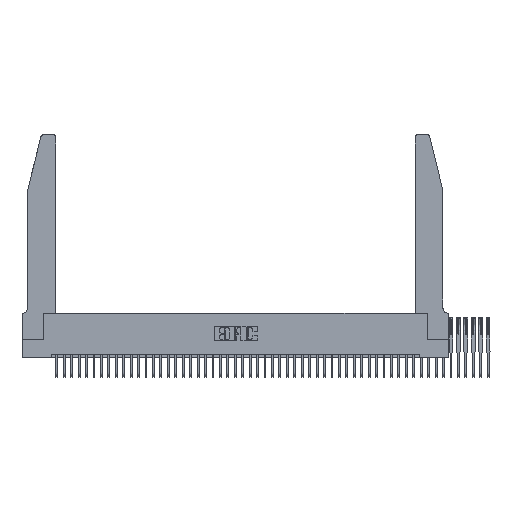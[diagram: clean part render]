
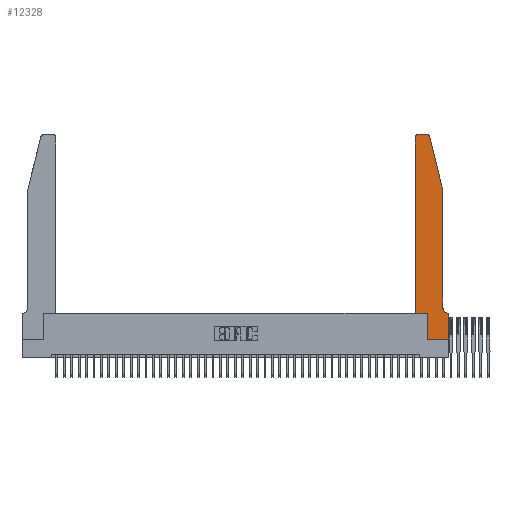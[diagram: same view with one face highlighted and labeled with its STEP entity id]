
A CAD part, top view. The second image highlights one B-rep face of the part: STEP entity #12328.
In plain terms, the highlighted face is planar.
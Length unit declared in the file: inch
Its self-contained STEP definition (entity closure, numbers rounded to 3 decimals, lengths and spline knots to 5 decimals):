
#178 = EDGE_CURVE ( 'NONE', #13072, #494, #8193, .T. ) ;
#361 = CARTESIAN_POINT ( 'NONE',  ( 0.0055, 0.42, 0. ) ) ;
#494 = VERTEX_POINT ( 'NONE', #31878 ) ;
#635 = CARTESIAN_POINT ( 'NONE',  ( 0.25487, 2.72718, 0. ) ) ;
#930 = VECTOR ( 'NONE', #30856, 39.37008 ) ;
#1835 = LINE ( 'NONE', #7803, #26412 ) ;
#2104 = CARTESIAN_POINT ( 'NONE',  ( 0., 0.35, 0. ) ) ;
#2577 = VERTEX_POINT ( 'NONE', #7879 ) ;
#2579 = ORIENTED_EDGE ( 'NONE', *, *, #7124, .F. ) ;
#2732 = CARTESIAN_POINT ( 'NONE',  ( 0.0755, 0.42, 0. ) ) ;
#2834 = EDGE_LOOP ( 'NONE', ( #19985, #33211, #2840, #29865, #11579, #32295, #10594, #4968, #27315, #2579, #9077, #7560 ) ) ;
#2840 = ORIENTED_EDGE ( 'NONE', *, *, #12280, .F. ) ;
#2904 = VERTEX_POINT ( 'NONE', #34921 ) ;
#3621 = DIRECTION ( 'NONE',  ( 0., 0., -1. ) ) ;
#3631 = VECTOR ( 'NONE', #8545, 39.37008 ) ;
#3675 = DIRECTION ( 'NONE',  ( -1., 0., 0. ) ) ;
#4968 = ORIENTED_EDGE ( 'NONE', *, *, #16838, .F. ) ;
#5735 = CARTESIAN_POINT ( 'NONE',  ( 0.2865, 0., 0. ) ) ;
#6922 = VERTEX_POINT ( 'NONE', #35473 ) ;
#7002 = VECTOR ( 'NONE', #38113, 39.37008 ) ;
#7124 = EDGE_CURVE ( 'NONE', #35716, #32932, #27854, .T. ) ;
#7560 = ORIENTED_EDGE ( 'NONE', *, *, #15237, .F. ) ;
#7798 = CIRCLE ( 'NONE', #17933, 0.03 ) ;
#7803 = CARTESIAN_POINT ( 'NONE',  ( 0.2605, 2.75, 0. ) ) ;
#7879 = CARTESIAN_POINT ( 'NONE',  ( 0.4205, 2.75, 0. ) ) ;
#8089 = CARTESIAN_POINT ( 'NONE',  ( 0.0755, 0.35, 0. ) ) ;
#8193 = LINE ( 'NONE', #30409, #32463 ) ;
#8531 = EDGE_CURVE ( 'NONE', #38510, #35024, #7798, .T. ) ;
#8545 = DIRECTION ( 'NONE',  ( 1., 0., 0. ) ) ;
#8669 = DIRECTION ( 'NONE',  ( 0., 0., 1. ) ) ;
#9077 = ORIENTED_EDGE ( 'NONE', *, *, #23521, .F. ) ;
#9122 = AXIS2_PLACEMENT_3D ( 'NONE', #2104, #8669, #30847 ) ;
#10409 = EDGE_CURVE ( 'NONE', #31535, #31510, #28615, .T. ) ;
#10594 = ORIENTED_EDGE ( 'NONE', *, *, #10409, .F. ) ;
#10720 = EDGE_CURVE ( 'NONE', #2577, #494, #25149, .T. ) ;
#11100 = DIRECTION ( 'NONE',  ( 0., 0., -1. ) ) ;
#11107 = DIRECTION ( 'NONE',  ( -1., 0., 0. ) ) ;
#11230 = EDGE_CURVE ( 'NONE', #32932, #6922, #30482, .T. ) ;
#11383 = DIRECTION ( 'NONE',  ( -1., 0., 0. ) ) ;
#11579 = ORIENTED_EDGE ( 'NONE', *, *, #178, .F. ) ;
#12280 = EDGE_CURVE ( 'NONE', #2577, #35024, #1835, .T. ) ;
#12328 = ADVANCED_FACE ( 'NONE', ( #32747 ), #27716, .F. ) ;
#13072 = VERTEX_POINT ( 'NONE', #37435 ) ;
#14738 = VECTOR ( 'NONE', #34578, 39.37008 ) ;
#15237 = EDGE_CURVE ( 'NONE', #2904, #31575, #20240, .T. ) ;
#16241 = CARTESIAN_POINT ( 'NONE',  ( 0., 0., 0. ) ) ;
#16657 = LINE ( 'NONE', #16241, #7002 ) ;
#16838 = EDGE_CURVE ( 'NONE', #6922, #31535, #16657, .T. ) ;
#16917 = DIRECTION ( 'NONE',  ( 0., -1., 0. ) ) ;
#17933 = AXIS2_PLACEMENT_3D ( 'NONE', #30034, #11100, #33162 ) ;
#19985 = ORIENTED_EDGE ( 'NONE', *, *, #29763, .F. ) ;
#20081 = CARTESIAN_POINT ( 'NONE',  ( 0.0755, 2., 0. ) ) ;
#20240 = LINE ( 'NONE', #20081, #28586 ) ;
#20271 = VECTOR ( 'NONE', #24283, 39.37008 ) ;
#21134 = CARTESIAN_POINT ( 'NONE',  ( 0.2865, 0.35, 0. ) ) ;
#21289 = CARTESIAN_POINT ( 'NONE',  ( 0.4505, 0.35, 0. ) ) ;
#22905 = CARTESIAN_POINT ( 'NONE',  ( 0.4205, 2.72, 0. ) ) ;
#22961 = DIRECTION ( 'NONE',  ( 0., 0., -1. ) ) ;
#23160 = CIRCLE ( 'NONE', #34618, 0.07 ) ;
#23359 = CARTESIAN_POINT ( 'NONE',  ( 0.284, 2.75, 0. ) ) ;
#23521 = EDGE_CURVE ( 'NONE', #31575, #35716, #23160, .T. ) ;
#23780 = AXIS2_PLACEMENT_3D ( 'NONE', #22905, #3621, #26029 ) ;
#24283 = DIRECTION ( 'NONE',  ( 0., 1., 0. ) ) ;
#24770 = CARTESIAN_POINT ( 'NONE',  ( 0.2865, 0.35, 0. ) ) ;
#24914 = VECTOR ( 'NONE', #11383, 39.37008 ) ;
#25149 = CIRCLE ( 'NONE', #23780, 0.03 ) ;
#26029 = DIRECTION ( 'NONE',  ( 1., 0., 0. ) ) ;
#26412 = VECTOR ( 'NONE', #11107, 39.37008 ) ;
#27315 = ORIENTED_EDGE ( 'NONE', *, *, #11230, .F. ) ;
#27716 = PLANE ( 'NONE',  #9122 ) ;
#27854 = LINE ( 'NONE', #8089, #24914 ) ;
#28462 = CARTESIAN_POINT ( 'NONE',  ( 0., 0., 0. ) ) ;
#28586 = VECTOR ( 'NONE', #16917, 39.37008 ) ;
#28615 = LINE ( 'NONE', #21134, #20271 ) ;
#29137 = LINE ( 'NONE', #21289, #3631 ) ;
#29763 = EDGE_CURVE ( 'NONE', #38510, #2904, #34833, .T. ) ;
#29865 = ORIENTED_EDGE ( 'NONE', *, *, #10720, .T. ) ;
#30034 = CARTESIAN_POINT ( 'NONE',  ( 0.284, 2.72, 0. ) ) ;
#30143 = CARTESIAN_POINT ( 'NONE',  ( 0.0055, 0.35, 0. ) ) ;
#30409 = CARTESIAN_POINT ( 'NONE',  ( 0.4505, 0.35, 0. ) ) ;
#30482 = LINE ( 'NONE', #28462, #14738 ) ;
#30847 = DIRECTION ( 'NONE',  ( 1., 0., 0. ) ) ;
#30856 = DIRECTION ( 'NONE',  ( -0.239, -0.971, 0. ) ) ;
#31510 = VERTEX_POINT ( 'NONE', #24770 ) ;
#31535 = VERTEX_POINT ( 'NONE', #5735 ) ;
#31575 = VERTEX_POINT ( 'NONE', #2732 ) ;
#31878 = CARTESIAN_POINT ( 'NONE',  ( 0.4505, 2.72, 0. ) ) ;
#32165 = CARTESIAN_POINT ( 'NONE',  ( 0., 0.35, 0. ) ) ;
#32295 = ORIENTED_EDGE ( 'NONE', *, *, #37046, .F. ) ;
#32463 = VECTOR ( 'NONE', #33281, 39.37008 ) ;
#32747 = FACE_OUTER_BOUND ( 'NONE', #2834, .T. ) ;
#32932 = VERTEX_POINT ( 'NONE', #32165 ) ;
#33162 = DIRECTION ( 'NONE',  ( 1., 0., 0. ) ) ;
#33211 = ORIENTED_EDGE ( 'NONE', *, *, #8531, .T. ) ;
#33281 = DIRECTION ( 'NONE',  ( 0., 1., 0. ) ) ;
#34578 = DIRECTION ( 'NONE',  ( 0., -1., 0. ) ) ;
#34618 = AXIS2_PLACEMENT_3D ( 'NONE', #361, #22961, #3675 ) ;
#34833 = LINE ( 'NONE', #40183, #930 ) ;
#34921 = CARTESIAN_POINT ( 'NONE',  ( 0.0755, 2., 0. ) ) ;
#35024 = VERTEX_POINT ( 'NONE', #23359 ) ;
#35473 = CARTESIAN_POINT ( 'NONE',  ( 0., 0., 0. ) ) ;
#35716 = VERTEX_POINT ( 'NONE', #30143 ) ;
#37046 = EDGE_CURVE ( 'NONE', #31510, #13072, #29137, .T. ) ;
#37435 = CARTESIAN_POINT ( 'NONE',  ( 0.4505, 0.35, 0. ) ) ;
#38113 = DIRECTION ( 'NONE',  ( 1., 0., 0. ) ) ;
#38510 = VERTEX_POINT ( 'NONE', #635 ) ;
#40183 = CARTESIAN_POINT ( 'NONE',  ( 0.0755, 2., 0. ) ) ;
